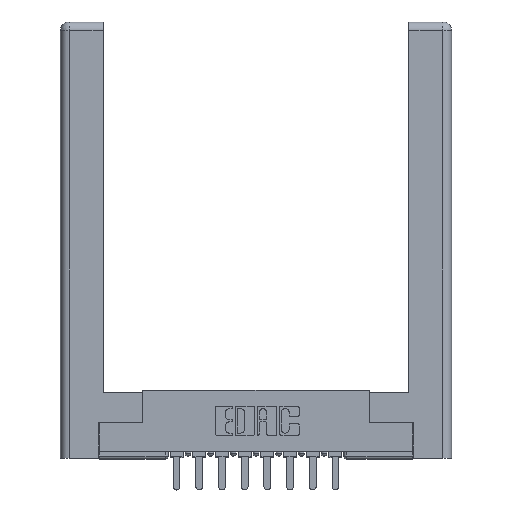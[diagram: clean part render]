
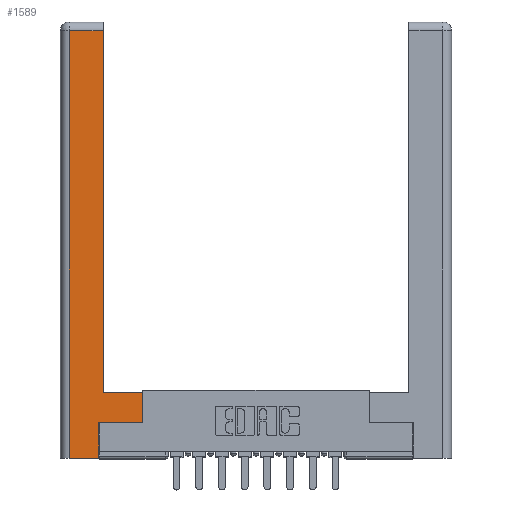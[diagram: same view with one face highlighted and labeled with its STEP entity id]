
A CAD part, top view. The second image highlights one B-rep face of the part: STEP entity #1589.
In plain terms, the highlighted planar face has unit normal (0, 0, 1).
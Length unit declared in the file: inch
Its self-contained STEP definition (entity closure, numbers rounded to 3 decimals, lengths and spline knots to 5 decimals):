
#38 = EDGE_CURVE ( 'NONE', #10067, #4344, #2678, .T. ) ;
#76 = VECTOR ( 'NONE', #10368, 39.37008 ) ;
#101 = EDGE_LOOP ( 'NONE', ( #7467, #1832, #14149, #11334, #8017, #7097, #4641, #1798 ) ) ;
#245 = EDGE_CURVE ( 'NONE', #9358, #10179, #13304, .T. ) ;
#274 = VERTEX_POINT ( 'NONE', #9527 ) ;
#350 = LINE ( 'NONE', #2956, #4730 ) ;
#851 = CARTESIAN_POINT ( 'NONE',  ( 0.265, 0., 0. ) ) ;
#919 = DIRECTION ( 'NONE',  ( -1., 0., 0. ) ) ;
#1340 = LINE ( 'NONE', #12315, #2384 ) ;
#1449 = LINE ( 'NONE', #8826, #3000 ) ;
#1553 = LINE ( 'NONE', #12003, #11656 ) ;
#1589 = ADVANCED_FACE ( 'NONE', ( #11494 ), #12013, .F. ) ;
#1798 = ORIENTED_EDGE ( 'NONE', *, *, #5375, .T. ) ;
#1832 = ORIENTED_EDGE ( 'NONE', *, *, #6034, .T. ) ;
#1834 = CARTESIAN_POINT ( 'NONE',  ( 0.295, 0.45, 0. ) ) ;
#2024 = DIRECTION ( 'NONE',  ( 0., 1., 0. ) ) ;
#2065 = EDGE_CURVE ( 'NONE', #10179, #274, #1553, .T. ) ;
#2384 = VECTOR ( 'NONE', #13528, 39.37008 ) ;
#2678 = LINE ( 'NONE', #4325, #6017 ) ;
#2956 = CARTESIAN_POINT ( 'NONE',  ( 0.565, 0.45, 0. ) ) ;
#3000 = VECTOR ( 'NONE', #7705, 39.37008 ) ;
#3046 = DIRECTION ( 'NONE',  ( 0., 0., -1. ) ) ;
#3060 = CARTESIAN_POINT ( 'NONE',  ( 0.295, 0.45, 0. ) ) ;
#3480 = AXIS2_PLACEMENT_3D ( 'NONE', #7564, #3046, #919 ) ;
#4188 = LINE ( 'NONE', #851, #10968 ) ;
#4325 = CARTESIAN_POINT ( 'NONE',  ( 0.0615, 0., 0. ) ) ;
#4344 = VERTEX_POINT ( 'NONE', #7951 ) ;
#4632 = LINE ( 'NONE', #3060, #9145 ) ;
#4641 = ORIENTED_EDGE ( 'NONE', *, *, #8148, .T. ) ;
#4730 = VECTOR ( 'NONE', #2024, 39.37008 ) ;
#4748 = CARTESIAN_POINT ( 'NONE',  ( 0.565, 0.45, 0. ) ) ;
#5375 = EDGE_CURVE ( 'NONE', #12237, #5899, #4632, .T. ) ;
#5899 = VERTEX_POINT ( 'NONE', #1834 ) ;
#6017 = VECTOR ( 'NONE', #14373, 39.37008 ) ;
#6034 = EDGE_CURVE ( 'NONE', #10769, #10067, #1449, .T. ) ;
#6122 = CARTESIAN_POINT ( 'NONE',  ( 0.265, 0., 0. ) ) ;
#6526 = CARTESIAN_POINT ( 'NONE',  ( 0.295, 2.94, 0. ) ) ;
#7097 = ORIENTED_EDGE ( 'NONE', *, *, #2065, .T. ) ;
#7467 = ORIENTED_EDGE ( 'NONE', *, *, #10353, .T. ) ;
#7564 = CARTESIAN_POINT ( 'NONE',  ( 0., 0., 0. ) ) ;
#7705 = DIRECTION ( 'NONE',  ( -1., 0., 0. ) ) ;
#7951 = CARTESIAN_POINT ( 'NONE',  ( 0.0615, 0., 0. ) ) ;
#8017 = ORIENTED_EDGE ( 'NONE', *, *, #245, .T. ) ;
#8148 = EDGE_CURVE ( 'NONE', #274, #12237, #350, .T. ) ;
#8826 = CARTESIAN_POINT ( 'NONE',  ( 0.0615, 2.94, 0. ) ) ;
#8918 = EDGE_CURVE ( 'NONE', #4344, #9358, #4188, .T. ) ;
#9145 = VECTOR ( 'NONE', #13147, 39.37008 ) ;
#9358 = VERTEX_POINT ( 'NONE', #6122 ) ;
#9527 = CARTESIAN_POINT ( 'NONE',  ( 0.565, 0.245, 0. ) ) ;
#9712 = DIRECTION ( 'NONE',  ( 1., 0., 0. ) ) ;
#10067 = VERTEX_POINT ( 'NONE', #10838 ) ;
#10179 = VERTEX_POINT ( 'NONE', #14006 ) ;
#10353 = EDGE_CURVE ( 'NONE', #5899, #10769, #1340, .T. ) ;
#10368 = DIRECTION ( 'NONE',  ( 0., 1., 0. ) ) ;
#10769 = VERTEX_POINT ( 'NONE', #6526 ) ;
#10838 = CARTESIAN_POINT ( 'NONE',  ( 0.0615, 2.94, 0. ) ) ;
#10968 = VECTOR ( 'NONE', #9712, 39.37008 ) ;
#11334 = ORIENTED_EDGE ( 'NONE', *, *, #8918, .T. ) ;
#11494 = FACE_OUTER_BOUND ( 'NONE', #101, .T. ) ;
#11656 = VECTOR ( 'NONE', #14239, 39.37008 ) ;
#12003 = CARTESIAN_POINT ( 'NONE',  ( 0.565, 0.245, 0. ) ) ;
#12013 = PLANE ( 'NONE',  #3480 ) ;
#12237 = VERTEX_POINT ( 'NONE', #4748 ) ;
#12315 = CARTESIAN_POINT ( 'NONE',  ( 0.295, 3., 0. ) ) ;
#12797 = CARTESIAN_POINT ( 'NONE',  ( 0.265, 0.245, 0. ) ) ;
#13147 = DIRECTION ( 'NONE',  ( -1., 0., 0. ) ) ;
#13304 = LINE ( 'NONE', #12797, #76 ) ;
#13528 = DIRECTION ( 'NONE',  ( 0., 1., 0. ) ) ;
#14006 = CARTESIAN_POINT ( 'NONE',  ( 0.265, 0.245, 0. ) ) ;
#14149 = ORIENTED_EDGE ( 'NONE', *, *, #38, .T. ) ;
#14239 = DIRECTION ( 'NONE',  ( 1., 0., 0. ) ) ;
#14373 = DIRECTION ( 'NONE',  ( 0., -1., 0. ) ) ;
